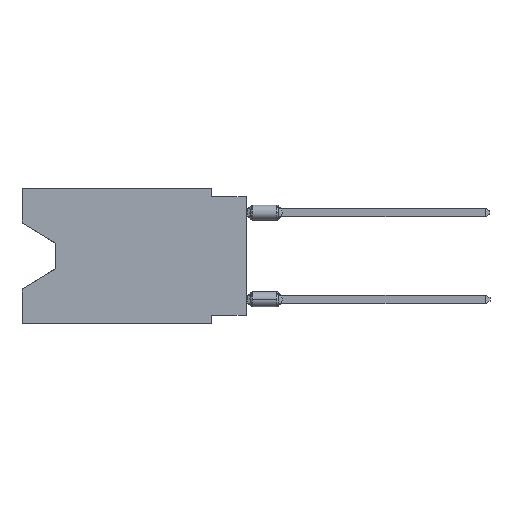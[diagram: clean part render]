
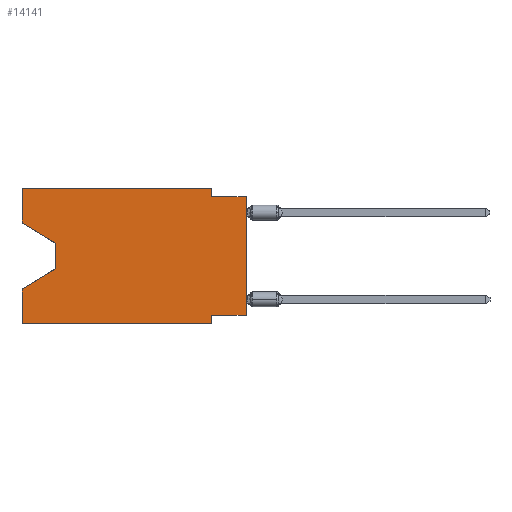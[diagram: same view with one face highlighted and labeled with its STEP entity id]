
A CAD part, left-side view. The second image highlights one B-rep face of the part: STEP entity #14141.
In plain terms, the highlighted planar face has unit normal (-1, 0, 0).
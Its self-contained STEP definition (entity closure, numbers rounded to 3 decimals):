
#169 = VECTOR ( 'NONE', #656, 1000. ) ;
#433 = CARTESIAN_POINT ( 'NONE',  ( 0., 16.383, -9.906 ) ) ;
#450 = VECTOR ( 'NONE', #14308, 1000. ) ;
#531 = LINE ( 'NONE', #17555, #13929 ) ;
#656 = DIRECTION ( 'NONE',  ( 0., 0., -1. ) ) ;
#972 = ORIENTED_EDGE ( 'NONE', *, *, #13531, .T. ) ;
#1151 = CARTESIAN_POINT ( 'NONE',  ( 0., 13.97, -5.893 ) ) ;
#1258 = CARTESIAN_POINT ( 'NONE',  ( 0., 0., -9.271 ) ) ;
#1338 = DIRECTION ( 'NONE',  ( 0., 0., -1. ) ) ;
#1421 = DIRECTION ( 'NONE',  ( 0., 0.855, -0.519 ) ) ;
#1773 = EDGE_LOOP ( 'NONE', ( #11825, #972, #9913, #15090, #18534, #9944, #15947, #11426, #3810, #11126, #2875, #18054 ) ) ;
#2267 = CARTESIAN_POINT ( 'NONE',  ( 0., 16.383, 0. ) ) ;
#2351 = LINE ( 'NONE', #5173, #169 ) ;
#2503 = VERTEX_POINT ( 'NONE', #5697 ) ;
#2751 = EDGE_CURVE ( 'NONE', #10328, #17332, #9635, .T. ) ;
#2819 = CARTESIAN_POINT ( 'NONE',  ( 0., 16.383, 0. ) ) ;
#2875 = ORIENTED_EDGE ( 'NONE', *, *, #17680, .F. ) ;
#2995 = VECTOR ( 'NONE', #10498, 1000. ) ;
#3160 = CARTESIAN_POINT ( 'NONE',  ( 0., 13.97, -5.893 ) ) ;
#3276 = CARTESIAN_POINT ( 'NONE',  ( 0., 2.54, -0.635 ) ) ;
#3767 = EDGE_CURVE ( 'NONE', #10371, #13316, #15335, .T. ) ;
#3810 = ORIENTED_EDGE ( 'NONE', *, *, #2751, .F. ) ;
#3812 = CARTESIAN_POINT ( 'NONE',  ( 0., 0., -0.635 ) ) ;
#3879 = EDGE_CURVE ( 'NONE', #10559, #17332, #14584, .T. ) ;
#4019 = DIRECTION ( 'NONE',  ( 0., -1., 0. ) ) ;
#4150 = EDGE_CURVE ( 'NONE', #10404, #17252, #6839, .T. ) ;
#4200 = LINE ( 'NONE', #16886, #14545 ) ;
#4506 = EDGE_CURVE ( 'NONE', #17603, #6083, #8407, .T. ) ;
#4644 = VECTOR ( 'NONE', #15907, 1000. ) ;
#4807 = EDGE_CURVE ( 'NONE', #2503, #10328, #2351, .T. ) ;
#4966 = VERTEX_POINT ( 'NONE', #18411 ) ;
#5118 = DIRECTION ( 'NONE',  ( 0., -1., 0. ) ) ;
#5173 = CARTESIAN_POINT ( 'NONE',  ( 0., 2.54, 0. ) ) ;
#5395 = CARTESIAN_POINT ( 'NONE',  ( 0., 13.97, -4.013 ) ) ;
#5697 = CARTESIAN_POINT ( 'NONE',  ( 0., 2.54, 0. ) ) ;
#5844 = VERTEX_POINT ( 'NONE', #7383 ) ;
#5996 = CARTESIAN_POINT ( 'NONE',  ( 0., 2.54, -9.906 ) ) ;
#6083 = VERTEX_POINT ( 'NONE', #18426 ) ;
#6111 = VECTOR ( 'NONE', #8908, 1000. ) ;
#6239 = VECTOR ( 'NONE', #5118, 1000. ) ;
#6478 = VECTOR ( 'NONE', #1421, 1000. ) ;
#6608 = CARTESIAN_POINT ( 'NONE',  ( 0., 16.383, 0. ) ) ;
#6839 = LINE ( 'NONE', #12391, #17286 ) ;
#7383 = CARTESIAN_POINT ( 'NONE',  ( 0., 2.54, -9.271 ) ) ;
#7505 = CARTESIAN_POINT ( 'NONE',  ( 0., 16.383, -2.546 ) ) ;
#8378 = CARTESIAN_POINT ( 'NONE',  ( 0., 16.383, 0. ) ) ;
#8407 = LINE ( 'NONE', #1151, #6478 ) ;
#8597 = EDGE_CURVE ( 'NONE', #10371, #4966, #13584, .T. ) ;
#8908 = DIRECTION ( 'NONE',  ( 0., -1., 0. ) ) ;
#9003 = CARTESIAN_POINT ( 'NONE',  ( 0., 16.383, 0. ) ) ;
#9635 = LINE ( 'NONE', #3812, #6239 ) ;
#9913 = ORIENTED_EDGE ( 'NONE', *, *, #4506, .T. ) ;
#9944 = ORIENTED_EDGE ( 'NONE', *, *, #17567, .F. ) ;
#10299 = LINE ( 'NONE', #9003, #6111 ) ;
#10328 = VERTEX_POINT ( 'NONE', #3276 ) ;
#10371 = VERTEX_POINT ( 'NONE', #7505 ) ;
#10404 = VERTEX_POINT ( 'NONE', #433 ) ;
#10498 = DIRECTION ( 'NONE',  ( 0., -0.855, -0.519 ) ) ;
#10559 = VERTEX_POINT ( 'NONE', #1258 ) ;
#10663 = VECTOR ( 'NONE', #10997, 1000. ) ;
#10671 = VECTOR ( 'NONE', #1338, 1000. ) ;
#10997 = DIRECTION ( 'NONE',  ( 0., 0., 1. ) ) ;
#11126 = ORIENTED_EDGE ( 'NONE', *, *, #4807, .F. ) ;
#11219 = LINE ( 'NONE', #5395, #10671 ) ;
#11426 = ORIENTED_EDGE ( 'NONE', *, *, #3879, .T. ) ;
#11825 = ORIENTED_EDGE ( 'NONE', *, *, #8597, .T. ) ;
#12391 = CARTESIAN_POINT ( 'NONE',  ( 0., 16.383, -9.906 ) ) ;
#12808 = CARTESIAN_POINT ( 'NONE',  ( 0., 0., -0.635 ) ) ;
#13163 = CARTESIAN_POINT ( 'NONE',  ( 0., 0., 0. ) ) ;
#13316 = VERTEX_POINT ( 'NONE', #6608 ) ;
#13531 = EDGE_CURVE ( 'NONE', #4966, #17603, #11219, .T. ) ;
#13584 = LINE ( 'NONE', #17642, #2995 ) ;
#13681 = EDGE_CURVE ( 'NONE', #10404, #6083, #17196, .T. ) ;
#13929 = VECTOR ( 'NONE', #17378, 1000. ) ;
#14141 = ADVANCED_FACE ( 'NONE', ( #15343 ), #15256, .F. ) ;
#14308 = DIRECTION ( 'NONE',  ( 0., 0., 1. ) ) ;
#14545 = VECTOR ( 'NONE', #18378, 1000. ) ;
#14584 = LINE ( 'NONE', #13163, #4644 ) ;
#15066 = DIRECTION ( 'NONE',  ( 1., 0., 0. ) ) ;
#15090 = ORIENTED_EDGE ( 'NONE', *, *, #13681, .F. ) ;
#15256 = PLANE ( 'NONE',  #16680 ) ;
#15335 = LINE ( 'NONE', #8378, #10663 ) ;
#15343 = FACE_OUTER_BOUND ( 'NONE', #1773, .T. ) ;
#15907 = DIRECTION ( 'NONE',  ( 0., 0., 1. ) ) ;
#15947 = ORIENTED_EDGE ( 'NONE', *, *, #17777, .F. ) ;
#16649 = DIRECTION ( 'NONE',  ( 0., 0., -1. ) ) ;
#16680 = AXIS2_PLACEMENT_3D ( 'NONE', #2267, #15066, #16649 ) ;
#16886 = CARTESIAN_POINT ( 'NONE',  ( 0., 2.54, -9.906 ) ) ;
#17196 = LINE ( 'NONE', #2819, #450 ) ;
#17252 = VERTEX_POINT ( 'NONE', #5996 ) ;
#17286 = VECTOR ( 'NONE', #4019, 1000. ) ;
#17332 = VERTEX_POINT ( 'NONE', #12808 ) ;
#17378 = DIRECTION ( 'NONE',  ( 0., 1., 0. ) ) ;
#17555 = CARTESIAN_POINT ( 'NONE',  ( 0., 0., -9.271 ) ) ;
#17567 = EDGE_CURVE ( 'NONE', #5844, #17252, #4200, .T. ) ;
#17603 = VERTEX_POINT ( 'NONE', #3160 ) ;
#17642 = CARTESIAN_POINT ( 'NONE',  ( 0., 16.383, -2.546 ) ) ;
#17680 = EDGE_CURVE ( 'NONE', #13316, #2503, #10299, .T. ) ;
#17777 = EDGE_CURVE ( 'NONE', #10559, #5844, #531, .T. ) ;
#18054 = ORIENTED_EDGE ( 'NONE', *, *, #3767, .F. ) ;
#18378 = DIRECTION ( 'NONE',  ( 0., 0., -1. ) ) ;
#18411 = CARTESIAN_POINT ( 'NONE',  ( 0., 13.97, -4.013 ) ) ;
#18426 = CARTESIAN_POINT ( 'NONE',  ( 0., 16.383, -7.36 ) ) ;
#18534 = ORIENTED_EDGE ( 'NONE', *, *, #4150, .T. ) ;
